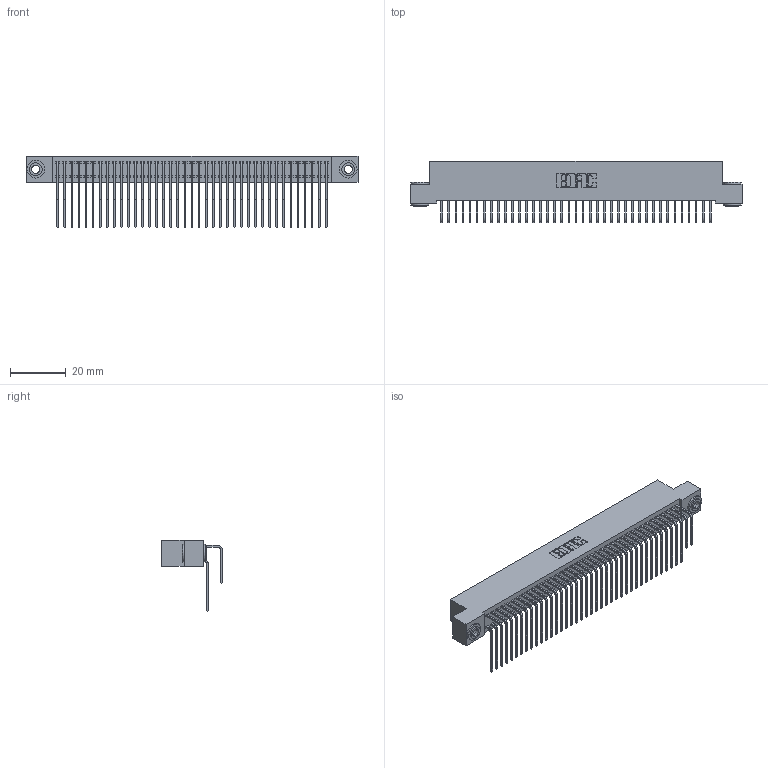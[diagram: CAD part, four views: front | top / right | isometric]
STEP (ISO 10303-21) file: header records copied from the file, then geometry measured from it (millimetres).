
FILE_DESCRIPTION (( 'STEP AP203' ), '1' );
FILE_NAME ('342-078-558-203.STEP', '2019-10-04T11:21:48', ( '' ), ( '' ), 'SwSTEP 2.0', 'SolidWorks 2016', '' );
FILE_SCHEMA (( 'CONFIG_CONTROL_DESIGN' ));
Length unit declared in the file: inch
Products named in the file (5): 342 Part_.156 TH; 345-292-001_558 559 Tail - 1; 345-292-001_558 Tail - 2; 342-250-002_345-250-002-102; 342-078-558-203
Assembly tree (81 placements, depth 2):
  342-078-558-203
    342 Part_.156 TH
    345-292-001_558 559 Tail - 1  x39
    345-292-001_558 Tail - 2  x39
    342-250-002_345-250-002-102  x2
Bounding box: 119.38 x 21.91 x 25.78 mm (x, y, z)
Volume: 11184.9 mm3; surface area: 20381.8 mm2
Topology: 81 solids, 81 shells, 4360 faces, 12933 edges, 8514 vertices
Faces by surface type: plane 3040, cylinder 1312, cone 8
Entity records: 27780 total; most frequent: CARTESIAN_POINT 4632, ORIENTED_EDGE 4510, DIRECTION 3977, EDGE_CURVE 2255, LINE 2063, VECTOR 2063, VERTEX_POINT 1498, AXIS2_PLACEMENT_3D 957
